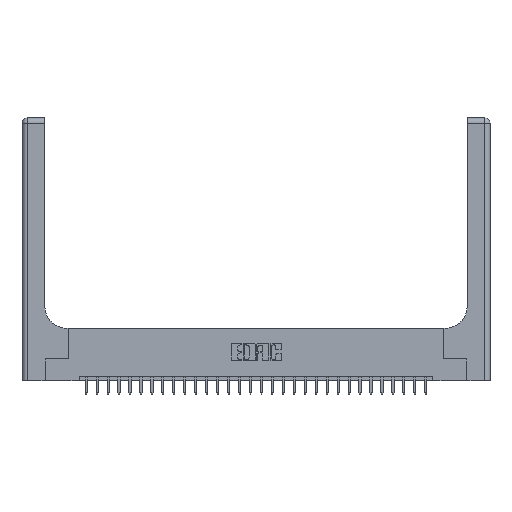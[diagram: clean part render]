
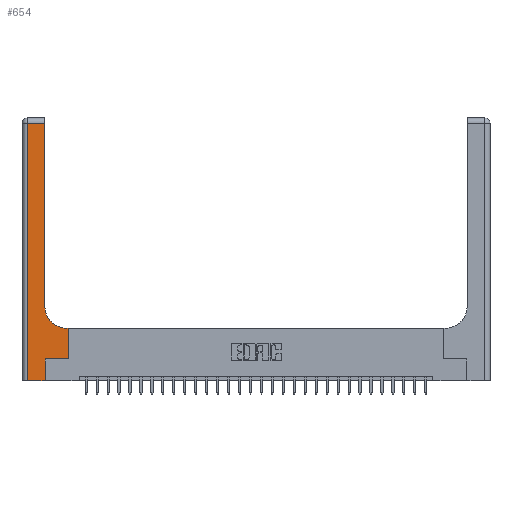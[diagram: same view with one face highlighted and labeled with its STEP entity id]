
A CAD part, top view. The second image highlights one B-rep face of the part: STEP entity #654.
In plain terms, the highlighted planar face has unit normal (0, 0, 1).
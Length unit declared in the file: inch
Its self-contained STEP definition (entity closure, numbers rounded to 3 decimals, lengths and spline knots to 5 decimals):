
#170 = DIRECTION ( 'NONE',  ( 0., -1., 0. ) ) ;
#345 = VECTOR ( 'NONE', #1661, 39.37008 ) ;
#357 = CARTESIAN_POINT ( 'NONE',  ( 0.06, 3., 0.37 ) ) ;
#654 = ADVANCED_FACE ( 'NONE', ( #25748 ), #14607, .F. ) ;
#1348 = DIRECTION ( 'NONE',  ( 1., 0., 0. ) ) ;
#1661 = DIRECTION ( 'NONE',  ( -1., 0., 0. ) ) ;
#1864 = DIRECTION ( 'NONE',  ( 0., 0., -1. ) ) ;
#1874 = LINE ( 'NONE', #6838, #9504 ) ;
#2231 = EDGE_CURVE ( 'NONE', #9376, #23964, #2746, .T. ) ;
#2746 = LINE ( 'NONE', #357, #13695 ) ;
#3189 = ORIENTED_EDGE ( 'NONE', *, *, #21049, .T. ) ;
#3323 = LINE ( 'NONE', #3884, #345 ) ;
#3626 = CARTESIAN_POINT ( 'NONE',  ( 0.51, 0.85, 0.37 ) ) ;
#3884 = CARTESIAN_POINT ( 'NONE',  ( 0.26, 0.6, 0.37 ) ) ;
#4254 = LINE ( 'NONE', #9771, #18839 ) ;
#4283 = ORIENTED_EDGE ( 'NONE', *, *, #24490, .T. ) ;
#4387 = EDGE_CURVE ( 'NONE', #11713, #14229, #13577, .T. ) ;
#5128 = EDGE_CURVE ( 'NONE', #25438, #9376, #4254, .T. ) ;
#5986 = EDGE_CURVE ( 'NONE', #14583, #11713, #1874, .T. ) ;
#6838 = CARTESIAN_POINT ( 'NONE',  ( 0.265, 0., 0.37 ) ) ;
#8593 = CARTESIAN_POINT ( 'NONE',  ( 0.265, 0.25, 0.37 ) ) ;
#8664 = CIRCLE ( 'NONE', #24741, 0.25 ) ;
#9182 = LINE ( 'NONE', #22549, #21772 ) ;
#9342 = CARTESIAN_POINT ( 'NONE',  ( 0.26, 3., 0.37 ) ) ;
#9376 = VERTEX_POINT ( 'NONE', #12807 ) ;
#9504 = VECTOR ( 'NONE', #10987, 39.37008 ) ;
#9771 = CARTESIAN_POINT ( 'NONE',  ( 0., 2.94, 0.37 ) ) ;
#10416 = EDGE_CURVE ( 'NONE', #22584, #12715, #3323, .T. ) ;
#10581 = ORIENTED_EDGE ( 'NONE', *, *, #25171, .T. ) ;
#10987 = DIRECTION ( 'NONE',  ( 0., 1., 0. ) ) ;
#11288 = VECTOR ( 'NONE', #23806, 39.37008 ) ;
#11536 = DIRECTION ( 'NONE',  ( 1., 0., 0. ) ) ;
#11713 = VERTEX_POINT ( 'NONE', #8593 ) ;
#11872 = DIRECTION ( 'NONE',  ( 0., 0., -1. ) ) ;
#12715 = VERTEX_POINT ( 'NONE', #25749 ) ;
#12717 = VECTOR ( 'NONE', #24190, 39.37008 ) ;
#12744 = CARTESIAN_POINT ( 'NONE',  ( 0.265, 0.25, 0.37 ) ) ;
#12807 = CARTESIAN_POINT ( 'NONE',  ( 0.06, 2.94, 0.37 ) ) ;
#13042 = ORIENTED_EDGE ( 'NONE', *, *, #21380, .T. ) ;
#13555 = ORIENTED_EDGE ( 'NONE', *, *, #2231, .T. ) ;
#13577 = LINE ( 'NONE', #12744, #15903 ) ;
#13695 = VECTOR ( 'NONE', #170, 39.37008 ) ;
#14229 = VERTEX_POINT ( 'NONE', #21364 ) ;
#14583 = VERTEX_POINT ( 'NONE', #18347 ) ;
#14607 = PLANE ( 'NONE',  #23360 ) ;
#14875 = CARTESIAN_POINT ( 'NONE',  ( 0.26, 0.85, 0.37 ) ) ;
#15903 = VECTOR ( 'NONE', #11536, 39.37008 ) ;
#17765 = ORIENTED_EDGE ( 'NONE', *, *, #10416, .T. ) ;
#18066 = CARTESIAN_POINT ( 'NONE',  ( 0., 3., 0.37 ) ) ;
#18347 = CARTESIAN_POINT ( 'NONE',  ( 0.265, 0., 0.37 ) ) ;
#18839 = VECTOR ( 'NONE', #24616, 39.37008 ) ;
#18925 = VERTEX_POINT ( 'NONE', #14875 ) ;
#19688 = CARTESIAN_POINT ( 'NONE',  ( 0.528, 0.25, 0.37 ) ) ;
#20243 = CARTESIAN_POINT ( 'NONE',  ( 0.528, 0.6, 0.37 ) ) ;
#20403 = ORIENTED_EDGE ( 'NONE', *, *, #5128, .T. ) ;
#20551 = ORIENTED_EDGE ( 'NONE', *, *, #5986, .T. ) ;
#21049 = EDGE_CURVE ( 'NONE', #12715, #18925, #8664, .T. ) ;
#21364 = CARTESIAN_POINT ( 'NONE',  ( 0.528, 0.25, 0.37 ) ) ;
#21380 = EDGE_CURVE ( 'NONE', #14229, #22584, #26231, .T. ) ;
#21772 = VECTOR ( 'NONE', #1348, 39.37008 ) ;
#22418 = DIRECTION ( 'NONE',  ( 1., 0., 0. ) ) ;
#22549 = CARTESIAN_POINT ( 'NONE',  ( 0., 0., 0.37 ) ) ;
#22584 = VERTEX_POINT ( 'NONE', #20243 ) ;
#23065 = ORIENTED_EDGE ( 'NONE', *, *, #4387, .T. ) ;
#23360 = AXIS2_PLACEMENT_3D ( 'NONE', #18066, #1864, #26491 ) ;
#23806 = DIRECTION ( 'NONE',  ( 0., 1., 0. ) ) ;
#23964 = VERTEX_POINT ( 'NONE', #27210 ) ;
#24190 = DIRECTION ( 'NONE',  ( 0., 1., 0. ) ) ;
#24490 = EDGE_CURVE ( 'NONE', #23964, #14583, #9182, .T. ) ;
#24616 = DIRECTION ( 'NONE',  ( -1., 0., 0. ) ) ;
#24741 = AXIS2_PLACEMENT_3D ( 'NONE', #3626, #11872, #22418 ) ;
#25171 = EDGE_CURVE ( 'NONE', #18925, #25438, #26679, .T. ) ;
#25438 = VERTEX_POINT ( 'NONE', #26407 ) ;
#25748 = FACE_OUTER_BOUND ( 'NONE', #26131, .T. ) ;
#25749 = CARTESIAN_POINT ( 'NONE',  ( 0.51, 0.6, 0.37 ) ) ;
#26131 = EDGE_LOOP ( 'NONE', ( #10581, #20403, #13555, #4283, #20551, #23065, #13042, #17765, #3189 ) ) ;
#26231 = LINE ( 'NONE', #19688, #11288 ) ;
#26407 = CARTESIAN_POINT ( 'NONE',  ( 0.26, 2.94, 0.37 ) ) ;
#26491 = DIRECTION ( 'NONE',  ( -1., 0., 0. ) ) ;
#26679 = LINE ( 'NONE', #9342, #12717 ) ;
#27210 = CARTESIAN_POINT ( 'NONE',  ( 0.06, 0., 0.37 ) ) ;
